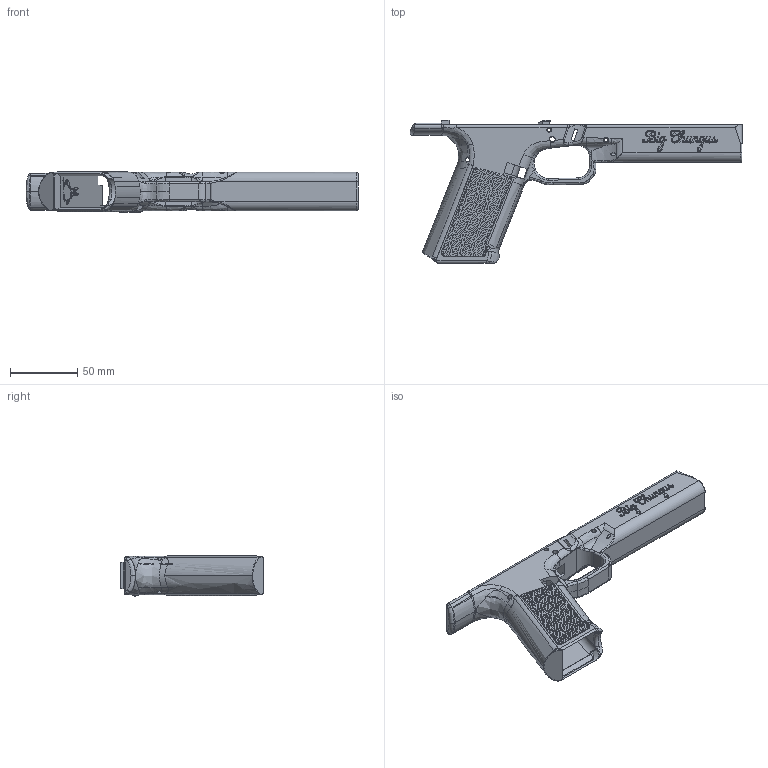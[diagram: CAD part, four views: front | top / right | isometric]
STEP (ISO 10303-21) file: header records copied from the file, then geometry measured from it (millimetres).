
FILE_DESCRIPTION(/* description */ (''),/* implementation_level */ '2;1');
FILE_NAME(/* name */ 'G17 Big Chungus.step',/* time_stamp */ '2021-04-09T08:53:18-06:00',/* author */ (''),/* organization */ (''),/* preprocessor_version */ 'ST-DEVELOPER v18.1',/* originating_system */ 'Autodesk Translation Framework v9.10.0.1330',/* authorisation */ '');
FILE_SCHEMA (('AUTOMOTIVE_DESIGN { 1 0 10303 214 3 1 1 }'));
Products named in the file (1): G17 Big Chungus
Bounding box: 247.28 x 106.5 x 30.34 mm (x, y, z)
Volume: 133294.7 mm3; surface area: 63107 mm2
Topology: 1 solids, 3 shells, 6398 faces, 18059 edges, 11901 vertices
Faces by surface type: bspline 4271, plane 1909, cylinder 153, torus 40, sphere 16, cone 9
Full cylindrical faces by diameter (mm): 2 x2, 3 x4, 3.2 x2, 4 x2, 9.55 x2
Entity records: 239778 total; most frequent: CARTESIAN_POINT 115606, ORIENTED_EDGE 36098, EDGE_CURVE 18049, DIRECTION 14341, VERTEX_POINT 11902, LINE 8875, VECTOR 8875, EDGE_LOOP 6677
